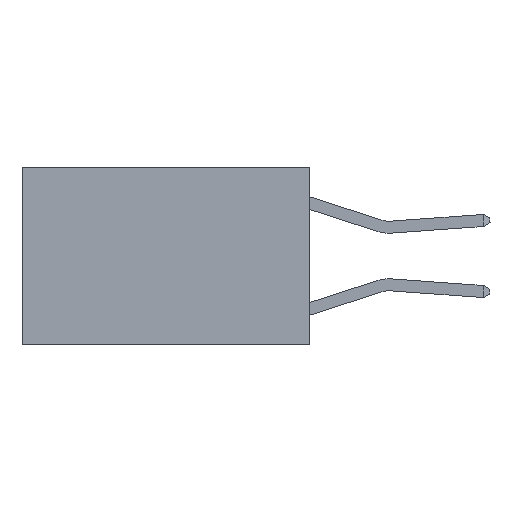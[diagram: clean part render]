
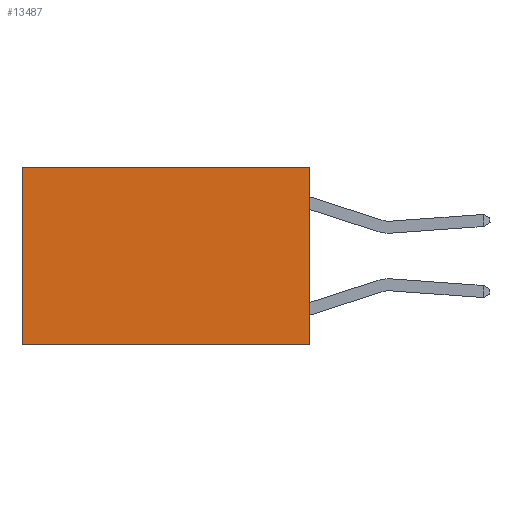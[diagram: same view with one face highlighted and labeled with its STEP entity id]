
A CAD part, left-side view. The second image highlights one B-rep face of the part: STEP entity #13487.
In plain terms, the highlighted planar face has unit normal (-1, 0, 0).
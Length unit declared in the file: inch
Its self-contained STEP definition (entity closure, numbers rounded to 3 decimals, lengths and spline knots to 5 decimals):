
#1737 = CARTESIAN_POINT ( 'NONE',  ( 0.2625, 0.6, 0. ) ) ;
#2981 = VECTOR ( 'NONE', #23042, 39.37008 ) ;
#3121 = VECTOR ( 'NONE', #14400, 39.37008 ) ;
#3255 = CARTESIAN_POINT ( 'NONE',  ( 0.2625, 0., 0. ) ) ;
#3584 = CARTESIAN_POINT ( 'NONE',  ( 0.2625, 0., 0. ) ) ;
#3612 = PLANE ( 'NONE',  #22066 ) ;
#6735 = CARTESIAN_POINT ( 'NONE',  ( 0.2625, 0., -0.37 ) ) ;
#9481 = ORIENTED_EDGE ( 'NONE', *, *, #15803, .F. ) ;
#9508 = VERTEX_POINT ( 'NONE', #1737 ) ;
#10293 = VERTEX_POINT ( 'NONE', #18031 ) ;
#10453 = LINE ( 'NONE', #16556, #2981 ) ;
#11683 = EDGE_CURVE ( 'NONE', #9508, #10293, #10453, .T. ) ;
#13487 = ADVANCED_FACE ( 'NONE', ( #13914 ), #3612, .F. ) ;
#13914 = FACE_OUTER_BOUND ( 'NONE', #15755, .T. ) ;
#14400 = DIRECTION ( 'NONE',  ( 0., 1., 0. ) ) ;
#14464 = DIRECTION ( 'NONE',  ( 1., 0., 0. ) ) ;
#15072 = VERTEX_POINT ( 'NONE', #6735 ) ;
#15332 = VECTOR ( 'NONE', #22292, 39.37008 ) ;
#15755 = EDGE_LOOP ( 'NONE', ( #19865, #9481, #25349, #21030 ) ) ;
#15803 = EDGE_CURVE ( 'NONE', #15072, #10293, #25270, .T. ) ;
#16556 = CARTESIAN_POINT ( 'NONE',  ( 0.2625, 0.6, 0. ) ) ;
#17686 = LINE ( 'NONE', #3584, #15332 ) ;
#18031 = CARTESIAN_POINT ( 'NONE',  ( 0.2625, 0.6, -0.37 ) ) ;
#18309 = CARTESIAN_POINT ( 'NONE',  ( 0.2625, 0., 0. ) ) ;
#18318 = CARTESIAN_POINT ( 'NONE',  ( 0.2625, 0., -0.37 ) ) ;
#19865 = ORIENTED_EDGE ( 'NONE', *, *, #11683, .T. ) ;
#20569 = EDGE_CURVE ( 'NONE', #23105, #15072, #26574, .T. ) ;
#21030 = ORIENTED_EDGE ( 'NONE', *, *, #22144, .T. ) ;
#22066 = AXIS2_PLACEMENT_3D ( 'NONE', #22448, #14464, #22177 ) ;
#22144 = EDGE_CURVE ( 'NONE', #23105, #9508, #17686, .T. ) ;
#22177 = DIRECTION ( 'NONE',  ( 0., 0., -1. ) ) ;
#22292 = DIRECTION ( 'NONE',  ( 0., 1., 0. ) ) ;
#22448 = CARTESIAN_POINT ( 'NONE',  ( 0.2625, 0., 0. ) ) ;
#22649 = DIRECTION ( 'NONE',  ( 0., 0., -1. ) ) ;
#23042 = DIRECTION ( 'NONE',  ( 0., 0., -1. ) ) ;
#23105 = VERTEX_POINT ( 'NONE', #3255 ) ;
#24357 = VECTOR ( 'NONE', #22649, 39.37008 ) ;
#25270 = LINE ( 'NONE', #18318, #3121 ) ;
#25349 = ORIENTED_EDGE ( 'NONE', *, *, #20569, .F. ) ;
#26574 = LINE ( 'NONE', #18309, #24357 ) ;
